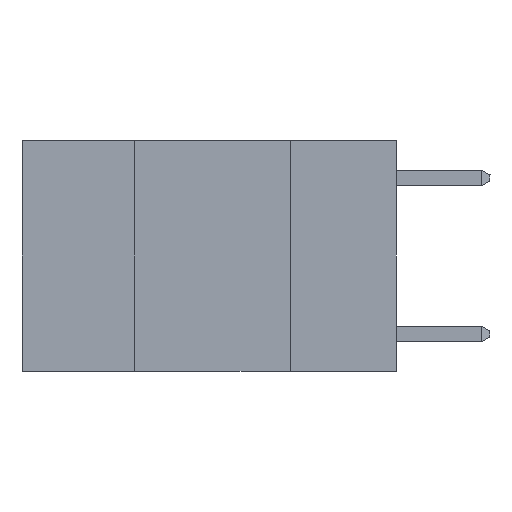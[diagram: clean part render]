
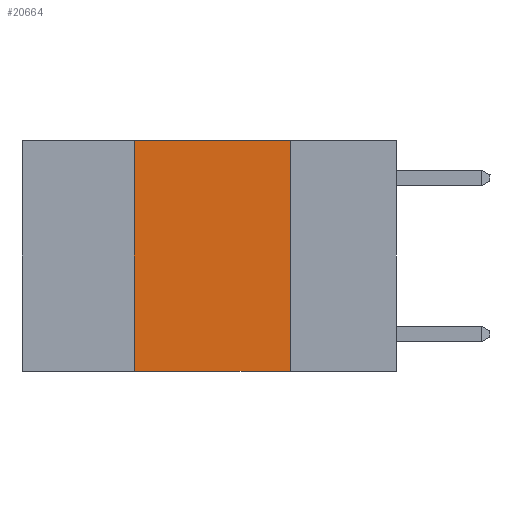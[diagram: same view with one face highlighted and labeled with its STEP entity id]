
A CAD part, left-side view. The second image highlights one B-rep face of the part: STEP entity #20664.
In plain terms, the highlighted planar face has unit normal (-1, 0, 0).
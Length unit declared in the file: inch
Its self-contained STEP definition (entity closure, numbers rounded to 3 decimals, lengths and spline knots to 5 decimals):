
#657 = EDGE_CURVE ( 'NONE', #11609, #12715, #4142, .T. ) ;
#1673 = ORIENTED_EDGE ( 'NONE', *, *, #25077, .T. ) ;
#1753 = VECTOR ( 'NONE', #12001, 39.37008 ) ;
#1865 = DIRECTION ( 'NONE',  ( 1., 0., 0. ) ) ;
#3266 = DIRECTION ( 'NONE',  ( 0., 0., -1. ) ) ;
#3411 = EDGE_CURVE ( 'NONE', #4062, #8933, #14721, .T. ) ;
#4062 = VERTEX_POINT ( 'NONE', #7358 ) ;
#4142 = LINE ( 'NONE', #11445, #19341 ) ;
#6328 = AXIS2_PLACEMENT_3D ( 'NONE', #7863, #1865, #15863 ) ;
#7358 = CARTESIAN_POINT ( 'NONE',  ( 0., 0.17, 0. ) ) ;
#7793 = CARTESIAN_POINT ( 'NONE',  ( 0., 0.17, -0.37 ) ) ;
#7863 = CARTESIAN_POINT ( 'NONE',  ( 0., 0.6, 0. ) ) ;
#8018 = FACE_OUTER_BOUND ( 'NONE', #20604, .T. ) ;
#8559 = ORIENTED_EDGE ( 'NONE', *, *, #657, .F. ) ;
#8933 = VERTEX_POINT ( 'NONE', #7793 ) ;
#9216 = CARTESIAN_POINT ( 'NONE',  ( 0., 0.17, 0. ) ) ;
#9368 = CARTESIAN_POINT ( 'NONE',  ( 0., 0.42, 0. ) ) ;
#9994 = CARTESIAN_POINT ( 'NONE',  ( 0., 0.6, 0. ) ) ;
#10667 = LINE ( 'NONE', #19766, #19916 ) ;
#11445 = CARTESIAN_POINT ( 'NONE',  ( 0., 0.42, 0. ) ) ;
#11609 = VERTEX_POINT ( 'NONE', #18158 ) ;
#12001 = DIRECTION ( 'NONE',  ( 0., -1., 0. ) ) ;
#12715 = VERTEX_POINT ( 'NONE', #9368 ) ;
#13470 = DIRECTION ( 'NONE',  ( 0., 0., 1. ) ) ;
#14303 = ORIENTED_EDGE ( 'NONE', *, *, #3411, .F. ) ;
#14721 = LINE ( 'NONE', #9216, #23918 ) ;
#15844 = DIRECTION ( 'NONE',  ( 0., -1., 0. ) ) ;
#15863 = DIRECTION ( 'NONE',  ( 0., 0., -1. ) ) ;
#16652 = ORIENTED_EDGE ( 'NONE', *, *, #19998, .F. ) ;
#17693 = LINE ( 'NONE', #9994, #1753 ) ;
#18158 = CARTESIAN_POINT ( 'NONE',  ( 0., 0.42, -0.37 ) ) ;
#19341 = VECTOR ( 'NONE', #13470, 39.37008 ) ;
#19766 = CARTESIAN_POINT ( 'NONE',  ( 0., 0.6, -0.37 ) ) ;
#19916 = VECTOR ( 'NONE', #15844, 39.37008 ) ;
#19998 = EDGE_CURVE ( 'NONE', #12715, #4062, #17693, .T. ) ;
#20604 = EDGE_LOOP ( 'NONE', ( #14303, #16652, #8559, #1673 ) ) ;
#20664 = ADVANCED_FACE ( 'NONE', ( #8018 ), #25570, .F. ) ;
#23918 = VECTOR ( 'NONE', #3266, 39.37008 ) ;
#25077 = EDGE_CURVE ( 'NONE', #11609, #8933, #10667, .T. ) ;
#25570 = PLANE ( 'NONE',  #6328 ) ;
